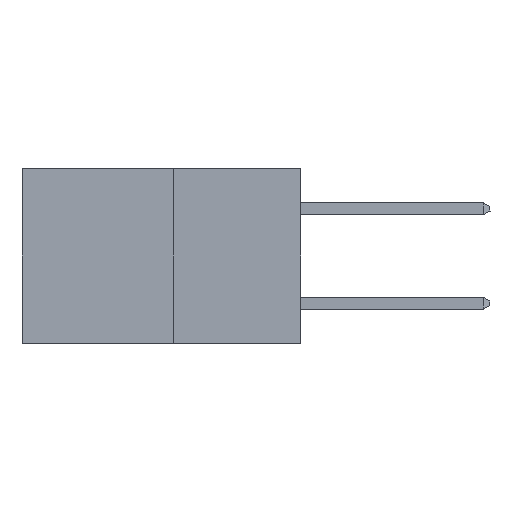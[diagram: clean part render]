
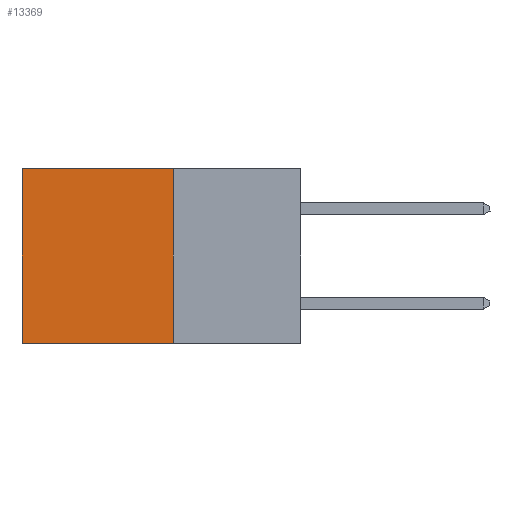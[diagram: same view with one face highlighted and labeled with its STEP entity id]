
A CAD part, left-side view. The second image highlights one B-rep face of the part: STEP entity #13369.
In plain terms, the highlighted planar face has unit normal (-1, 0, 0).
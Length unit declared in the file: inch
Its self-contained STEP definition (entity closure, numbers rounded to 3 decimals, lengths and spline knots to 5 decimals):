
#64 = PLANE ( 'NONE',  #2878 ) ;
#1344 = ORIENTED_EDGE ( 'NONE', *, *, #10179, .F. ) ;
#1778 = DIRECTION ( 'NONE',  ( 0., 0., -1. ) ) ;
#1989 = DIRECTION ( 'NONE',  ( 0., 1., 0. ) ) ;
#2194 = FACE_OUTER_BOUND ( 'NONE', #15773, .T. ) ;
#2803 = CARTESIAN_POINT ( 'NONE',  ( 0.277, 0.27, -0.37 ) ) ;
#2878 = AXIS2_PLACEMENT_3D ( 'NONE', #11724, #3670, #13051 ) ;
#2959 = VERTEX_POINT ( 'NONE', #13195 ) ;
#3174 = EDGE_CURVE ( 'NONE', #6423, #8600, #11305, .T. ) ;
#3295 = EDGE_CURVE ( 'NONE', #2959, #8600, #6096, .T. ) ;
#3438 = EDGE_CURVE ( 'NONE', #16272, #2959, #10674, .T. ) ;
#3670 = DIRECTION ( 'NONE',  ( 1., 0., 0. ) ) ;
#3897 = VECTOR ( 'NONE', #14701, 39.37008 ) ;
#6096 = LINE ( 'NONE', #6248, #12735 ) ;
#6248 = CARTESIAN_POINT ( 'NONE',  ( 0.277, 0.59, -0.37 ) ) ;
#6423 = VERTEX_POINT ( 'NONE', #12958 ) ;
#6657 = LINE ( 'NONE', #13857, #7514 ) ;
#7309 = DIRECTION ( 'NONE',  ( 0., 0., -1. ) ) ;
#7379 = VECTOR ( 'NONE', #1989, 39.37008 ) ;
#7514 = VECTOR ( 'NONE', #7309, 39.37008 ) ;
#8600 = VERTEX_POINT ( 'NONE', #14789 ) ;
#9068 = CARTESIAN_POINT ( 'NONE',  ( 0.277, 0.27, 0. ) ) ;
#9450 = ORIENTED_EDGE ( 'NONE', *, *, #3295, .T. ) ;
#10179 = EDGE_CURVE ( 'NONE', #16272, #6423, #6657, .T. ) ;
#10674 = LINE ( 'NONE', #9068, #3897 ) ;
#11305 = LINE ( 'NONE', #2803, #7379 ) ;
#11724 = CARTESIAN_POINT ( 'NONE',  ( 0.277, 0.27, -0.37 ) ) ;
#12735 = VECTOR ( 'NONE', #1778, 39.37008 ) ;
#12949 = ORIENTED_EDGE ( 'NONE', *, *, #3438, .T. ) ;
#12958 = CARTESIAN_POINT ( 'NONE',  ( 0.277, 0.27, -0.37 ) ) ;
#13051 = DIRECTION ( 'NONE',  ( 0., 0., -1. ) ) ;
#13195 = CARTESIAN_POINT ( 'NONE',  ( 0.277, 0.59, 0. ) ) ;
#13369 = ADVANCED_FACE ( 'NONE', ( #2194 ), #64, .F. ) ;
#13427 = CARTESIAN_POINT ( 'NONE',  ( 0.277, 0.27, 0. ) ) ;
#13753 = ORIENTED_EDGE ( 'NONE', *, *, #3174, .F. ) ;
#13857 = CARTESIAN_POINT ( 'NONE',  ( 0.277, 0.27, -0.37 ) ) ;
#14701 = DIRECTION ( 'NONE',  ( 0., 1., 0. ) ) ;
#14789 = CARTESIAN_POINT ( 'NONE',  ( 0.277, 0.59, -0.37 ) ) ;
#15773 = EDGE_LOOP ( 'NONE', ( #9450, #13753, #1344, #12949 ) ) ;
#16272 = VERTEX_POINT ( 'NONE', #13427 ) ;
